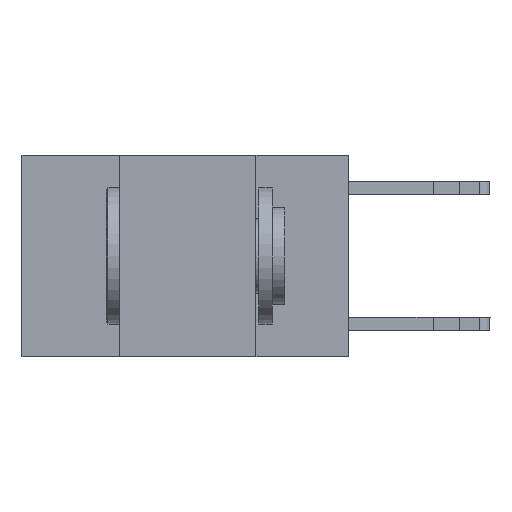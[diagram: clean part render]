
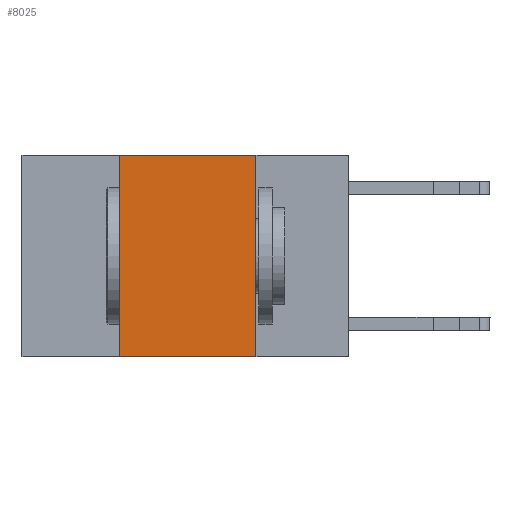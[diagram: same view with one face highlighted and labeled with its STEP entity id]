
A CAD part, left-side view. The second image highlights one B-rep face of the part: STEP entity #8025.
In plain terms, the highlighted planar face has unit normal (-1, 0, 0).
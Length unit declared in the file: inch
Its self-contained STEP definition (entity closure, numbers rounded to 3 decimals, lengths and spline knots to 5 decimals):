
#1362 = PLANE ( 'NONE',  #7145 ) ;
#1582 = DIRECTION ( 'NONE',  ( 0., 0., -1. ) ) ;
#1837 = LINE ( 'NONE', #13956, #17876 ) ;
#2211 = DIRECTION ( 'NONE',  ( 0., -1., 0. ) ) ;
#3566 = CARTESIAN_POINT ( 'NONE',  ( 0., 0.42, 0. ) ) ;
#3672 = EDGE_LOOP ( 'NONE', ( #18492, #6213, #14034, #5703 ) ) ;
#4125 = EDGE_CURVE ( 'NONE', #4489, #16063, #5311, .T. ) ;
#4141 = LINE ( 'NONE', #5373, #17949 ) ;
#4354 = FACE_OUTER_BOUND ( 'NONE', #3672, .T. ) ;
#4489 = VERTEX_POINT ( 'NONE', #10031 ) ;
#5311 = LINE ( 'NONE', #14818, #16844 ) ;
#5373 = CARTESIAN_POINT ( 'NONE',  ( 0., 0.6, 0. ) ) ;
#5703 = ORIENTED_EDGE ( 'NONE', *, *, #4125, .T. ) ;
#5797 = CARTESIAN_POINT ( 'NONE',  ( 0., 0.17, -0.37 ) ) ;
#6213 = ORIENTED_EDGE ( 'NONE', *, *, #8358, .F. ) ;
#7145 = AXIS2_PLACEMENT_3D ( 'NONE', #15626, #18707, #1582 ) ;
#8025 = ADVANCED_FACE ( 'NONE', ( #4354 ), #1362, .F. ) ;
#8143 = DIRECTION ( 'NONE',  ( 0., 0., -1. ) ) ;
#8358 = EDGE_CURVE ( 'NONE', #12683, #10220, #4141, .T. ) ;
#8433 = CARTESIAN_POINT ( 'NONE',  ( 0., 0.42, 0. ) ) ;
#8946 = DIRECTION ( 'NONE',  ( 0., 0., 1. ) ) ;
#10031 = CARTESIAN_POINT ( 'NONE',  ( 0., 0.42, -0.37 ) ) ;
#10220 = VERTEX_POINT ( 'NONE', #20024 ) ;
#10282 = VECTOR ( 'NONE', #8946, 39.37008 ) ;
#10429 = DIRECTION ( 'NONE',  ( 0., -1., 0. ) ) ;
#12683 = VERTEX_POINT ( 'NONE', #3566 ) ;
#12822 = EDGE_CURVE ( 'NONE', #4489, #12683, #17641, .T. ) ;
#13956 = CARTESIAN_POINT ( 'NONE',  ( 0., 0.17, 0. ) ) ;
#14034 = ORIENTED_EDGE ( 'NONE', *, *, #12822, .F. ) ;
#14818 = CARTESIAN_POINT ( 'NONE',  ( 0., 0.6, -0.37 ) ) ;
#15006 = EDGE_CURVE ( 'NONE', #10220, #16063, #1837, .T. ) ;
#15626 = CARTESIAN_POINT ( 'NONE',  ( 0., 0.6, 0. ) ) ;
#16063 = VERTEX_POINT ( 'NONE', #5797 ) ;
#16844 = VECTOR ( 'NONE', #2211, 39.37008 ) ;
#17641 = LINE ( 'NONE', #8433, #10282 ) ;
#17876 = VECTOR ( 'NONE', #8143, 39.37008 ) ;
#17949 = VECTOR ( 'NONE', #10429, 39.37008 ) ;
#18492 = ORIENTED_EDGE ( 'NONE', *, *, #15006, .F. ) ;
#18707 = DIRECTION ( 'NONE',  ( 1., 0., 0. ) ) ;
#20024 = CARTESIAN_POINT ( 'NONE',  ( 0., 0.17, 0. ) ) ;
